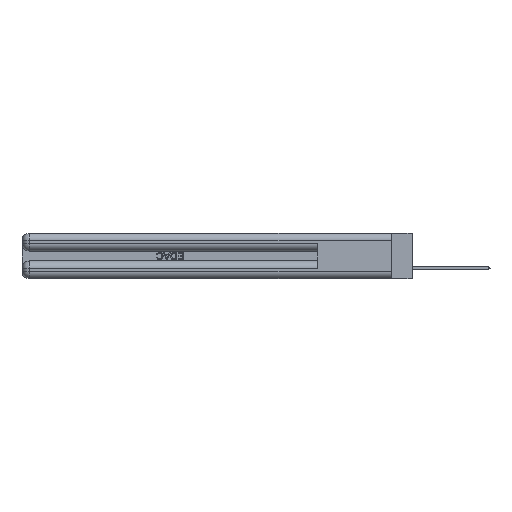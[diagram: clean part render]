
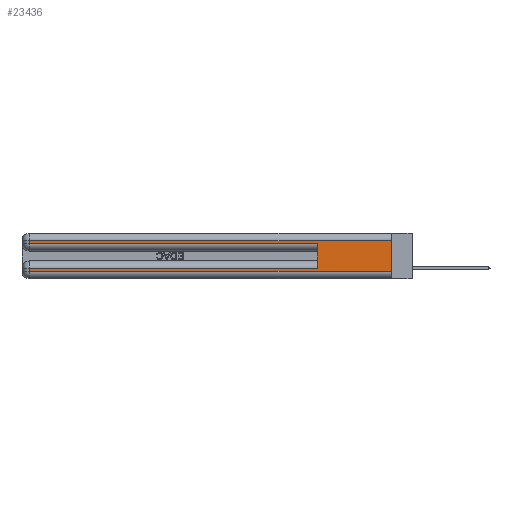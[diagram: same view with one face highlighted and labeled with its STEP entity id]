
A CAD part, left-side view. The second image highlights one B-rep face of the part: STEP entity #23436.
In plain terms, the highlighted planar face has unit normal (-1, 0, 0).
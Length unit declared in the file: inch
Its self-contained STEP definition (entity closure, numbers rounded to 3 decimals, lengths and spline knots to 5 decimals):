
#105 = CARTESIAN_POINT ( 'NONE',  ( 0., 0., 0.06 ) ) ;
#412 = EDGE_CURVE ( 'NONE', #10959, #20495, #39923, .T. ) ;
#1045 = VECTOR ( 'NONE', #31372, 39.37008 ) ;
#1440 = CARTESIAN_POINT ( 'NONE',  ( 0., 2.94, 0.37 ) ) ;
#3870 = VECTOR ( 'NONE', #7615, 39.37008 ) ;
#5298 = ORIENTED_EDGE ( 'NONE', *, *, #10458, .F. ) ;
#5486 = DIRECTION ( 'NONE',  ( 0., 0., -1. ) ) ;
#5621 = LINE ( 'NONE', #11296, #3870 ) ;
#5916 = DIRECTION ( 'NONE',  ( 1., 0., 0. ) ) ;
#7615 = DIRECTION ( 'NONE',  ( 0., -1., 0. ) ) ;
#8089 = EDGE_CURVE ( 'NONE', #43790, #30917, #43006, .T. ) ;
#8329 = CARTESIAN_POINT ( 'NONE',  ( 0., 0., 0.085 ) ) ;
#9460 = ORIENTED_EDGE ( 'NONE', *, *, #16146, .T. ) ;
#9653 = CARTESIAN_POINT ( 'NONE',  ( 0., 2.94, 0.085 ) ) ;
#10017 = CARTESIAN_POINT ( 'NONE',  ( 0., 2.94, 0.06 ) ) ;
#10458 = EDGE_CURVE ( 'NONE', #18738, #39391, #27968, .T. ) ;
#10488 = ORIENTED_EDGE ( 'NONE', *, *, #39496, .T. ) ;
#10959 = VERTEX_POINT ( 'NONE', #9653 ) ;
#11173 = EDGE_LOOP ( 'NONE', ( #5298, #9460, #21040, #27895, #30320, #10488, #24051, #35713 ) ) ;
#11296 = CARTESIAN_POINT ( 'NONE',  ( 0., 0., 0.285 ) ) ;
#14533 = CARTESIAN_POINT ( 'NONE',  ( 0., 0.6, 0.145 ) ) ;
#14788 = LINE ( 'NONE', #42947, #33713 ) ;
#16146 = EDGE_CURVE ( 'NONE', #18738, #43790, #19382, .T. ) ;
#17747 = EDGE_CURVE ( 'NONE', #34355, #37459, #30530, .T. ) ;
#18612 = CARTESIAN_POINT ( 'NONE',  ( 0., 0., 0.31 ) ) ;
#18738 = VERTEX_POINT ( 'NONE', #18612 ) ;
#19382 = LINE ( 'NONE', #37640, #43191 ) ;
#20453 = VECTOR ( 'NONE', #37559, 39.37008 ) ;
#20495 = VERTEX_POINT ( 'NONE', #10017 ) ;
#21040 = ORIENTED_EDGE ( 'NONE', *, *, #8089, .T. ) ;
#21088 = CARTESIAN_POINT ( 'NONE',  ( 0., 2.94, 0.37 ) ) ;
#21462 = AXIS2_PLACEMENT_3D ( 'NONE', #29704, #5916, #30178 ) ;
#23278 = VECTOR ( 'NONE', #31977, 39.37008 ) ;
#23436 = ADVANCED_FACE ( 'NONE', ( #42611 ), #47682, .F. ) ;
#24051 = ORIENTED_EDGE ( 'NONE', *, *, #412, .T. ) ;
#26575 = CARTESIAN_POINT ( 'NONE',  ( 0., 0., 0.37 ) ) ;
#27863 = DIRECTION ( 'NONE',  ( 0., 0., -1. ) ) ;
#27895 = ORIENTED_EDGE ( 'NONE', *, *, #43097, .T. ) ;
#27968 = LINE ( 'NONE', #26575, #29210 ) ;
#29210 = VECTOR ( 'NONE', #5486, 39.37008 ) ;
#29704 = CARTESIAN_POINT ( 'NONE',  ( 0., 0., 0.37 ) ) ;
#30178 = DIRECTION ( 'NONE',  ( 0., 0., -1. ) ) ;
#30320 = ORIENTED_EDGE ( 'NONE', *, *, #17747, .F. ) ;
#30530 = LINE ( 'NONE', #14533, #20453 ) ;
#30917 = VERTEX_POINT ( 'NONE', #39501 ) ;
#31372 = DIRECTION ( 'NONE',  ( 0., 1., 0. ) ) ;
#31977 = DIRECTION ( 'NONE',  ( 0., 0., -1. ) ) ;
#32032 = LINE ( 'NONE', #8329, #1045 ) ;
#33713 = VECTOR ( 'NONE', #43296, 39.37008 ) ;
#34355 = VERTEX_POINT ( 'NONE', #37003 ) ;
#34409 = DIRECTION ( 'NONE',  ( 0., 1., 0. ) ) ;
#35713 = ORIENTED_EDGE ( 'NONE', *, *, #37971, .T. ) ;
#37003 = CARTESIAN_POINT ( 'NONE',  ( 0., 0.6, 0.085 ) ) ;
#37118 = VECTOR ( 'NONE', #27863, 39.37008 ) ;
#37459 = VERTEX_POINT ( 'NONE', #40099 ) ;
#37559 = DIRECTION ( 'NONE',  ( 0., 0., 1. ) ) ;
#37640 = CARTESIAN_POINT ( 'NONE',  ( 0., 0., 0.31 ) ) ;
#37971 = EDGE_CURVE ( 'NONE', #20495, #39391, #14788, .T. ) ;
#39391 = VERTEX_POINT ( 'NONE', #105 ) ;
#39496 = EDGE_CURVE ( 'NONE', #34355, #10959, #32032, .T. ) ;
#39501 = CARTESIAN_POINT ( 'NONE',  ( 0., 2.94, 0.285 ) ) ;
#39898 = CARTESIAN_POINT ( 'NONE',  ( 0., 2.94, 0.31 ) ) ;
#39923 = LINE ( 'NONE', #21088, #23278 ) ;
#40099 = CARTESIAN_POINT ( 'NONE',  ( 0., 0.6, 0.285 ) ) ;
#42611 = FACE_OUTER_BOUND ( 'NONE', #11173, .T. ) ;
#42947 = CARTESIAN_POINT ( 'NONE',  ( 0., 0., 0.06 ) ) ;
#43006 = LINE ( 'NONE', #1440, #37118 ) ;
#43097 = EDGE_CURVE ( 'NONE', #30917, #37459, #5621, .T. ) ;
#43191 = VECTOR ( 'NONE', #34409, 39.37008 ) ;
#43296 = DIRECTION ( 'NONE',  ( 0., -1., 0. ) ) ;
#43790 = VERTEX_POINT ( 'NONE', #39898 ) ;
#47682 = PLANE ( 'NONE',  #21462 ) ;
